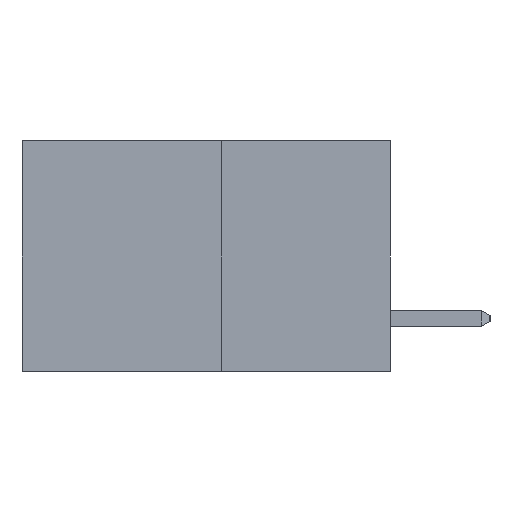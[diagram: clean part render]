
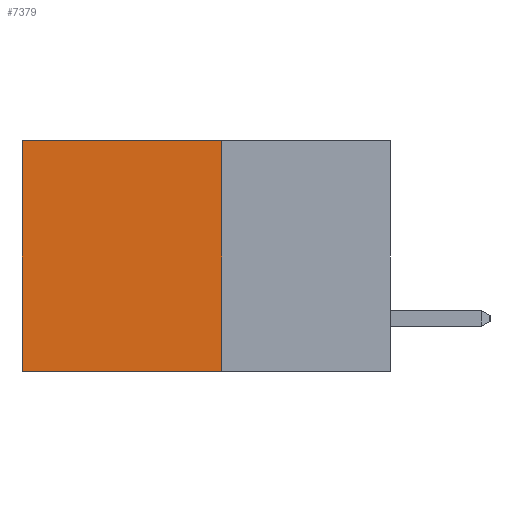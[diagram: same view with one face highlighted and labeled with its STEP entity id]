
A CAD part, left-side view. The second image highlights one B-rep face of the part: STEP entity #7379.
In plain terms, the highlighted planar face has unit normal (-1, 0, 0).
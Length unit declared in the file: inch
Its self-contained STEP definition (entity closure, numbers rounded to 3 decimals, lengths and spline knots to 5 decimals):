
#95 = VERTEX_POINT ( 'NONE', #9012 ) ;
#1421 = CARTESIAN_POINT ( 'NONE',  ( 0.277, 0.27, -0.37 ) ) ;
#1449 = FACE_OUTER_BOUND ( 'NONE', #4908, .T. ) ;
#1768 = CARTESIAN_POINT ( 'NONE',  ( 0.277, 0.27, -0.37 ) ) ;
#1946 = ORIENTED_EDGE ( 'NONE', *, *, #7999, .F. ) ;
#2052 = VERTEX_POINT ( 'NONE', #10758 ) ;
#2082 = VERTEX_POINT ( 'NONE', #10908 ) ;
#2287 = DIRECTION ( 'NONE',  ( 0., 1., 0. ) ) ;
#2766 = VECTOR ( 'NONE', #9553, 39.37008 ) ;
#3445 = EDGE_CURVE ( 'NONE', #8511, #2082, #11002, .T. ) ;
#3476 = CARTESIAN_POINT ( 'NONE',  ( 0.277, 0.27, 0. ) ) ;
#3865 = VECTOR ( 'NONE', #8348, 39.37008 ) ;
#3893 = CARTESIAN_POINT ( 'NONE',  ( 0.277, 0.27, 0. ) ) ;
#3909 = ORIENTED_EDGE ( 'NONE', *, *, #7069, .F. ) ;
#4084 = AXIS2_PLACEMENT_3D ( 'NONE', #11271, #11553, #11015 ) ;
#4169 = LINE ( 'NONE', #1768, #3865 ) ;
#4599 = PLANE ( 'NONE',  #4084 ) ;
#4787 = VECTOR ( 'NONE', #2287, 39.37008 ) ;
#4908 = EDGE_LOOP ( 'NONE', ( #8624, #3909, #1946, #6227 ) ) ;
#5866 = VECTOR ( 'NONE', #6029, 39.37008 ) ;
#6029 = DIRECTION ( 'NONE',  ( 0., 1., 0. ) ) ;
#6227 = ORIENTED_EDGE ( 'NONE', *, *, #3445, .T. ) ;
#7069 = EDGE_CURVE ( 'NONE', #95, #2052, #11683, .T. ) ;
#7379 = ADVANCED_FACE ( 'NONE', ( #1449 ), #4599, .F. ) ;
#7999 = EDGE_CURVE ( 'NONE', #8511, #95, #4169, .T. ) ;
#8348 = DIRECTION ( 'NONE',  ( 0., 0., -1. ) ) ;
#8511 = VERTEX_POINT ( 'NONE', #3476 ) ;
#8624 = ORIENTED_EDGE ( 'NONE', *, *, #9660, .T. ) ;
#9012 = CARTESIAN_POINT ( 'NONE',  ( 0.277, 0.27, -0.37 ) ) ;
#9517 = CARTESIAN_POINT ( 'NONE',  ( 0.277, 0.59, -0.37 ) ) ;
#9553 = DIRECTION ( 'NONE',  ( 0., 0., -1. ) ) ;
#9660 = EDGE_CURVE ( 'NONE', #2082, #2052, #10389, .T. ) ;
#10389 = LINE ( 'NONE', #9517, #2766 ) ;
#10758 = CARTESIAN_POINT ( 'NONE',  ( 0.277, 0.59, -0.37 ) ) ;
#10908 = CARTESIAN_POINT ( 'NONE',  ( 0.277, 0.59, 0. ) ) ;
#11002 = LINE ( 'NONE', #3893, #5866 ) ;
#11015 = DIRECTION ( 'NONE',  ( 0., 0., -1. ) ) ;
#11271 = CARTESIAN_POINT ( 'NONE',  ( 0.277, 0.27, -0.37 ) ) ;
#11553 = DIRECTION ( 'NONE',  ( 1., 0., 0. ) ) ;
#11683 = LINE ( 'NONE', #1421, #4787 ) ;
